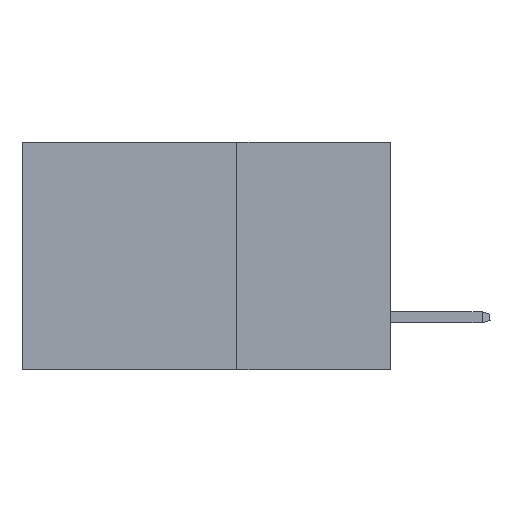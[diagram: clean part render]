
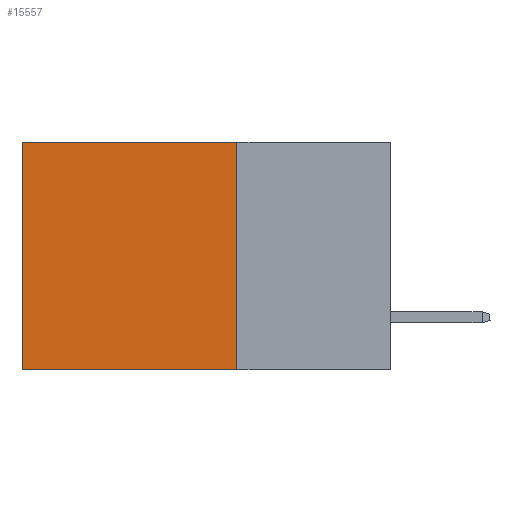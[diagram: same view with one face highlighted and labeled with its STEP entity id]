
A CAD part, left-side view. The second image highlights one B-rep face of the part: STEP entity #15557.
In plain terms, the highlighted planar face has unit normal (-1, 0, 0).
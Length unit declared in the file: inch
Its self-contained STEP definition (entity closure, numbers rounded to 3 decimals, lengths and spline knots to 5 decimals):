
#336 = ORIENTED_EDGE ( 'NONE', *, *, #524, .T. ) ;
#507 = CARTESIAN_POINT ( 'NONE',  ( 0.2875, 0.25, -0.37 ) ) ;
#524 = EDGE_CURVE ( 'NONE', #10988, #2953, #29411, .T. ) ;
#686 = AXIS2_PLACEMENT_3D ( 'NONE', #8933, #21126, #18138 ) ;
#2473 = EDGE_CURVE ( 'NONE', #32663, #10988, #8335, .T. ) ;
#2953 = VERTEX_POINT ( 'NONE', #38479 ) ;
#3046 = ORIENTED_EDGE ( 'NONE', *, *, #2473, .T. ) ;
#4850 = DIRECTION ( 'NONE',  ( 0., 0., -1. ) ) ;
#5353 = VERTEX_POINT ( 'NONE', #507 ) ;
#7761 = CARTESIAN_POINT ( 'NONE',  ( 0.2875, 0.25, 0. ) ) ;
#8335 = LINE ( 'NONE', #7761, #11546 ) ;
#8933 = CARTESIAN_POINT ( 'NONE',  ( 0.2875, 0.25, 0. ) ) ;
#10155 = CARTESIAN_POINT ( 'NONE',  ( 0.2875, 0.25, 0. ) ) ;
#10988 = VERTEX_POINT ( 'NONE', #37221 ) ;
#11381 = EDGE_LOOP ( 'NONE', ( #336, #18894, #37256, #3046 ) ) ;
#11546 = VECTOR ( 'NONE', #29330, 39.37008 ) ;
#11956 = PLANE ( 'NONE',  #686 ) ;
#14488 = VECTOR ( 'NONE', #4850, 39.37008 ) ;
#15557 = ADVANCED_FACE ( 'NONE', ( #39334 ), #11956, .F. ) ;
#16252 = DIRECTION ( 'NONE',  ( 0., 1., 0. ) ) ;
#18138 = DIRECTION ( 'NONE',  ( 0., 0., -1. ) ) ;
#18427 = CARTESIAN_POINT ( 'NONE',  ( 0.2875, 0.25, 0. ) ) ;
#18894 = ORIENTED_EDGE ( 'NONE', *, *, #29200, .F. ) ;
#21126 = DIRECTION ( 'NONE',  ( 1., 0., 0. ) ) ;
#21230 = VECTOR ( 'NONE', #31741, 39.37008 ) ;
#22207 = VECTOR ( 'NONE', #16252, 39.37008 ) ;
#26376 = LINE ( 'NONE', #34424, #22207 ) ;
#29200 = EDGE_CURVE ( 'NONE', #5353, #2953, #26376, .T. ) ;
#29330 = DIRECTION ( 'NONE',  ( 0., 1., 0. ) ) ;
#29411 = LINE ( 'NONE', #32429, #14488 ) ;
#31741 = DIRECTION ( 'NONE',  ( 0., 0., -1. ) ) ;
#32429 = CARTESIAN_POINT ( 'NONE',  ( 0.2875, 0.6, 0. ) ) ;
#32663 = VERTEX_POINT ( 'NONE', #18427 ) ;
#34424 = CARTESIAN_POINT ( 'NONE',  ( 0.2875, 0.25, -0.37 ) ) ;
#34946 = LINE ( 'NONE', #10155, #21230 ) ;
#35619 = EDGE_CURVE ( 'NONE', #32663, #5353, #34946, .T. ) ;
#37221 = CARTESIAN_POINT ( 'NONE',  ( 0.2875, 0.6, 0. ) ) ;
#37256 = ORIENTED_EDGE ( 'NONE', *, *, #35619, .F. ) ;
#38479 = CARTESIAN_POINT ( 'NONE',  ( 0.2875, 0.6, -0.37 ) ) ;
#39334 = FACE_OUTER_BOUND ( 'NONE', #11381, .T. ) ;
